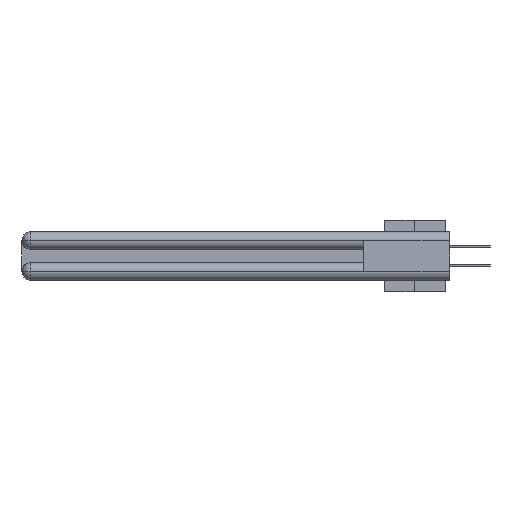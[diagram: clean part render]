
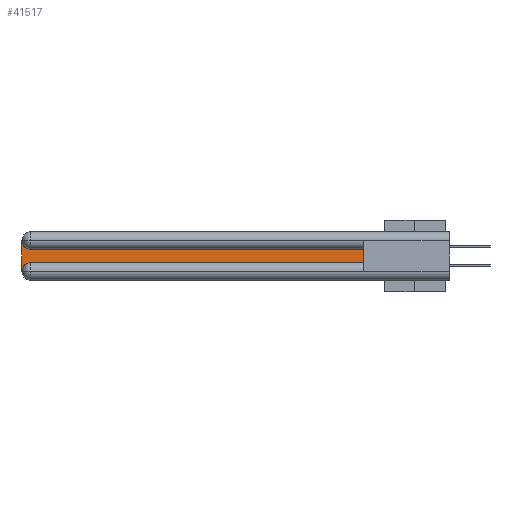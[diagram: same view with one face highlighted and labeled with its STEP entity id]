
A CAD part, left-side view. The second image highlights one B-rep face of the part: STEP entity #41517.
In plain terms, the highlighted planar face has unit normal (-1, 0, 0).
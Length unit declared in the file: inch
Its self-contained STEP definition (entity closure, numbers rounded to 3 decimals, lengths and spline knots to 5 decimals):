
#1185 = VERTEX_POINT ( 'NONE', #12985 ) ;
#1931 = CARTESIAN_POINT ( 'NONE',  ( 0.075, 2.94, -0.1225 ) ) ;
#3460 = EDGE_CURVE ( 'NONE', #15284, #39331, #37420, .T. ) ;
#5519 = DIRECTION ( 'NONE',  ( 0., 0., -1. ) ) ;
#7254 = DIRECTION ( 'NONE',  ( 1., 0., 0. ) ) ;
#7403 = CARTESIAN_POINT ( 'NONE',  ( 0.075, 2.94, -0.2775 ) ) ;
#8344 = CARTESIAN_POINT ( 'NONE',  ( 0.075, 0.6, -0.1225 ) ) ;
#8750 = VERTEX_POINT ( 'NONE', #17605 ) ;
#9912 = PLANE ( 'NONE',  #28149 ) ;
#12985 = CARTESIAN_POINT ( 'NONE',  ( 0.075, 0.6, -0.1225 ) ) ;
#14739 = DIRECTION ( 'NONE',  ( 0., 0., -1. ) ) ;
#15284 = VERTEX_POINT ( 'NONE', #31799 ) ;
#15346 = DIRECTION ( 'NONE',  ( 0., 0., -1. ) ) ;
#17211 = CARTESIAN_POINT ( 'NONE',  ( 0.075, 3., -0.1225 ) ) ;
#17605 = CARTESIAN_POINT ( 'NONE',  ( 0.075, 3., -0.0625 ) ) ;
#19678 = CIRCLE ( 'NONE', #39864, 0.06 ) ;
#21253 = ORIENTED_EDGE ( 'NONE', *, *, #31585, .T. ) ;
#21645 = EDGE_CURVE ( 'NONE', #39331, #38130, #26409, .T. ) ;
#22013 = DIRECTION ( 'NONE',  ( 0., 0., 1. ) ) ;
#22022 = LINE ( 'NONE', #33799, #40546 ) ;
#23267 = DIRECTION ( 'NONE',  ( 0., 1., 0. ) ) ;
#23923 = ORIENTED_EDGE ( 'NONE', *, *, #40759, .T. ) ;
#25336 = VECTOR ( 'NONE', #22013, 39.37008 ) ;
#25466 = VERTEX_POINT ( 'NONE', #1931 ) ;
#26372 = ORIENTED_EDGE ( 'NONE', *, *, #21645, .T. ) ;
#26409 = LINE ( 'NONE', #32044, #30428 ) ;
#27866 = DIRECTION ( 'NONE',  ( 0., 0., -1. ) ) ;
#28149 = AXIS2_PLACEMENT_3D ( 'NONE', #17211, #35512, #5519 ) ;
#28493 = DIRECTION ( 'NONE',  ( 0., -1., 0. ) ) ;
#29094 = VECTOR ( 'NONE', #23267, 39.37008 ) ;
#30305 = ORIENTED_EDGE ( 'NONE', *, *, #33231, .T. ) ;
#30428 = VECTOR ( 'NONE', #28493, 39.37008 ) ;
#31585 = EDGE_CURVE ( 'NONE', #8750, #15284, #22022, .T. ) ;
#31799 = CARTESIAN_POINT ( 'NONE',  ( 0.075, 3., -0.2775 ) ) ;
#31890 = CARTESIAN_POINT ( 'NONE',  ( 0.075, 2.94, -0.2175 ) ) ;
#32044 = CARTESIAN_POINT ( 'NONE',  ( 0.075, 0.6, -0.2175 ) ) ;
#33113 = LINE ( 'NONE', #8344, #29094 ) ;
#33231 = EDGE_CURVE ( 'NONE', #38130, #1185, #35148, .T. ) ;
#33799 = CARTESIAN_POINT ( 'NONE',  ( 0.075, 3., -0.2175 ) ) ;
#34966 = CARTESIAN_POINT ( 'NONE',  ( 0.075, 2.94, -0.0625 ) ) ;
#35148 = LINE ( 'NONE', #43885, #25336 ) ;
#35512 = DIRECTION ( 'NONE',  ( 1., 0., 0. ) ) ;
#36749 = ORIENTED_EDGE ( 'NONE', *, *, #3460, .T. ) ;
#37420 = CIRCLE ( 'NONE', #46219, 0.06 ) ;
#37684 = FACE_OUTER_BOUND ( 'NONE', #41434, .T. ) ;
#38130 = VERTEX_POINT ( 'NONE', #43074 ) ;
#38738 = DIRECTION ( 'NONE',  ( 1., 0., 0. ) ) ;
#39330 = EDGE_CURVE ( 'NONE', #25466, #8750, #19678, .T. ) ;
#39331 = VERTEX_POINT ( 'NONE', #31890 ) ;
#39401 = ORIENTED_EDGE ( 'NONE', *, *, #39330, .T. ) ;
#39864 = AXIS2_PLACEMENT_3D ( 'NONE', #34966, #38738, #27866 ) ;
#40546 = VECTOR ( 'NONE', #15346, 39.37008 ) ;
#40759 = EDGE_CURVE ( 'NONE', #1185, #25466, #33113, .T. ) ;
#41434 = EDGE_LOOP ( 'NONE', ( #23923, #39401, #21253, #36749, #26372, #30305 ) ) ;
#41517 = ADVANCED_FACE ( 'NONE', ( #37684 ), #9912, .F. ) ;
#43074 = CARTESIAN_POINT ( 'NONE',  ( 0.075, 0.6, -0.2175 ) ) ;
#43885 = CARTESIAN_POINT ( 'NONE',  ( 0.075, 0.6, -0.2175 ) ) ;
#46219 = AXIS2_PLACEMENT_3D ( 'NONE', #7403, #7254, #14739 ) ;
